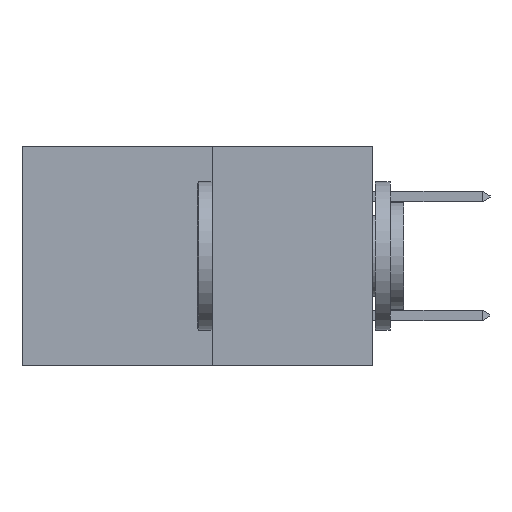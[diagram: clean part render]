
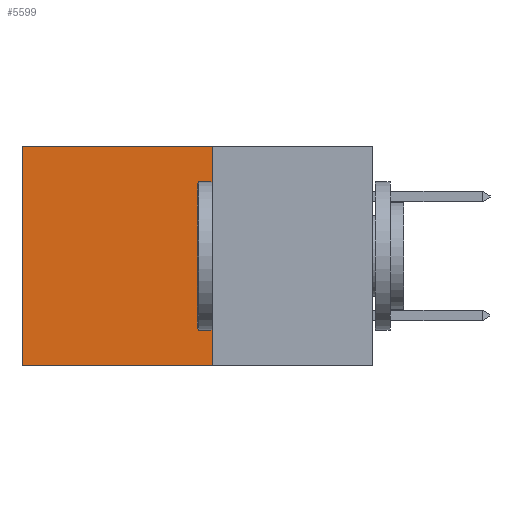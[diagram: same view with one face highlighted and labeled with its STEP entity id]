
A CAD part, left-side view. The second image highlights one B-rep face of the part: STEP entity #5599.
In plain terms, the highlighted planar face has unit normal (-1, 0, 0).
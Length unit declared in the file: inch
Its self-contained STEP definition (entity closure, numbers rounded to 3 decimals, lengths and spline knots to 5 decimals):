
#428 = LINE ( 'NONE', #6693, #4715 ) ;
#790 = DIRECTION ( 'NONE',  ( 0., 1., 0. ) ) ;
#1794 = EDGE_CURVE ( 'NONE', #2912, #9124, #8442, .T. ) ;
#2081 = EDGE_CURVE ( 'NONE', #9251, #9124, #9188, .T. ) ;
#2413 = DIRECTION ( 'NONE',  ( 0., 0., -1. ) ) ;
#2414 = DIRECTION ( 'NONE',  ( 1., 0., 0. ) ) ;
#2439 = CARTESIAN_POINT ( 'NONE',  ( 0.277, 0.27, -0.37 ) ) ;
#2450 = PLANE ( 'NONE',  #4589 ) ;
#2578 = CARTESIAN_POINT ( 'NONE',  ( 0.277, 0.27, 0. ) ) ;
#2707 = LINE ( 'NONE', #6153, #7130 ) ;
#2912 = VERTEX_POINT ( 'NONE', #3465 ) ;
#2942 = VECTOR ( 'NONE', #9519, 39.37008 ) ;
#3465 = CARTESIAN_POINT ( 'NONE',  ( 0.277, 0.27, -0.37 ) ) ;
#3690 = DIRECTION ( 'NONE',  ( 0., 0., -1. ) ) ;
#3707 = ORIENTED_EDGE ( 'NONE', *, *, #2081, .T. ) ;
#4589 = AXIS2_PLACEMENT_3D ( 'NONE', #2439, #2414, #2413 ) ;
#4715 = VECTOR ( 'NONE', #790, 39.37008 ) ;
#5524 = ORIENTED_EDGE ( 'NONE', *, *, #8460, .T. ) ;
#5599 = ADVANCED_FACE ( 'NONE', ( #6194 ), #2450, .F. ) ;
#5601 = VERTEX_POINT ( 'NONE', #2578 ) ;
#6017 = EDGE_LOOP ( 'NONE', ( #3707, #8177, #9069, #5524 ) ) ;
#6153 = CARTESIAN_POINT ( 'NONE',  ( 0.277, 0.27, -0.37 ) ) ;
#6194 = FACE_OUTER_BOUND ( 'NONE', #6017, .T. ) ;
#6294 = VECTOR ( 'NONE', #8075, 39.37008 ) ;
#6693 = CARTESIAN_POINT ( 'NONE',  ( 0.277, 0.27, 0. ) ) ;
#7130 = VECTOR ( 'NONE', #3690, 39.37008 ) ;
#7550 = CARTESIAN_POINT ( 'NONE',  ( 0.277, 0.59, 0. ) ) ;
#7577 = CARTESIAN_POINT ( 'NONE',  ( 0.277, 0.59, -0.37 ) ) ;
#8075 = DIRECTION ( 'NONE',  ( 0., 1., 0. ) ) ;
#8177 = ORIENTED_EDGE ( 'NONE', *, *, #1794, .F. ) ;
#8319 = CARTESIAN_POINT ( 'NONE',  ( 0.277, 0.27, -0.37 ) ) ;
#8442 = LINE ( 'NONE', #8319, #6294 ) ;
#8460 = EDGE_CURVE ( 'NONE', #5601, #9251, #428, .T. ) ;
#9069 = ORIENTED_EDGE ( 'NONE', *, *, #9464, .F. ) ;
#9124 = VERTEX_POINT ( 'NONE', #9782 ) ;
#9188 = LINE ( 'NONE', #7577, #2942 ) ;
#9251 = VERTEX_POINT ( 'NONE', #7550 ) ;
#9464 = EDGE_CURVE ( 'NONE', #5601, #2912, #2707, .T. ) ;
#9519 = DIRECTION ( 'NONE',  ( 0., 0., -1. ) ) ;
#9782 = CARTESIAN_POINT ( 'NONE',  ( 0.277, 0.59, -0.37 ) ) ;
